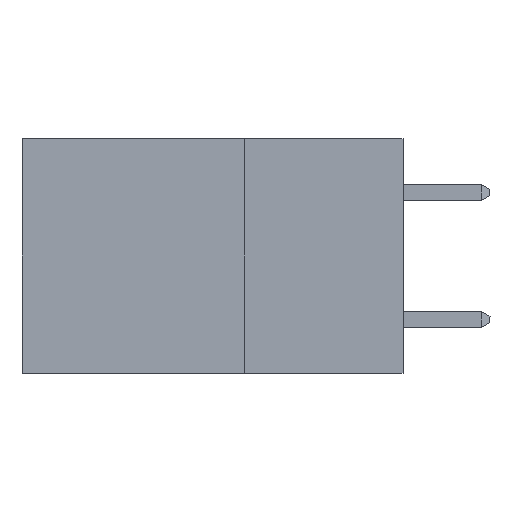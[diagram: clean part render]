
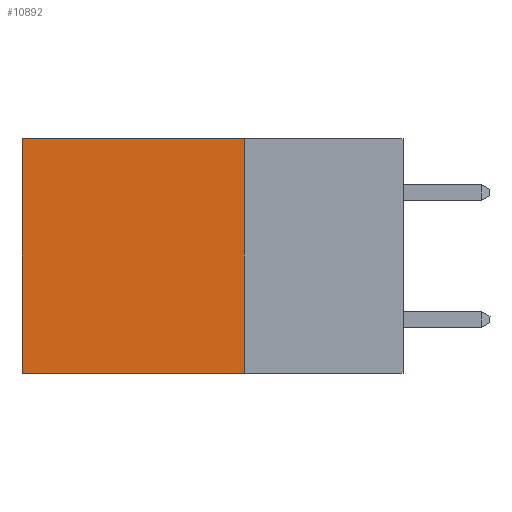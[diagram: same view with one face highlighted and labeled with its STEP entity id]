
A CAD part, left-side view. The second image highlights one B-rep face of the part: STEP entity #10892.
In plain terms, the highlighted planar face has unit normal (-1, 0, 0).
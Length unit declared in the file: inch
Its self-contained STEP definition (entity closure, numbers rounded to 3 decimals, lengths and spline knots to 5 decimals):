
#157 = ORIENTED_EDGE ( 'NONE', *, *, #10039, .F. ) ;
#158 = LINE ( 'NONE', #3170, #5974 ) ;
#489 = VERTEX_POINT ( 'NONE', #4031 ) ;
#647 = LINE ( 'NONE', #12323, #5846 ) ;
#1345 = DIRECTION ( 'NONE',  ( 0., 1., 0. ) ) ;
#1523 = CARTESIAN_POINT ( 'NONE',  ( 0.2875, 0.6, 0. ) ) ;
#1695 = VECTOR ( 'NONE', #12266, 39.37008 ) ;
#1858 = CARTESIAN_POINT ( 'NONE',  ( 0.2875, 0.25, 0. ) ) ;
#2393 = VECTOR ( 'NONE', #1345, 39.37008 ) ;
#2487 = VERTEX_POINT ( 'NONE', #4806 ) ;
#3170 = CARTESIAN_POINT ( 'NONE',  ( 0.2875, 0.25, 0. ) ) ;
#3178 = VERTEX_POINT ( 'NONE', #1523 ) ;
#3682 = ORIENTED_EDGE ( 'NONE', *, *, #5398, .T. ) ;
#3708 = DIRECTION ( 'NONE',  ( 1., 0., 0. ) ) ;
#4031 = CARTESIAN_POINT ( 'NONE',  ( 0.2875, 0.6, -0.37 ) ) ;
#4665 = FACE_OUTER_BOUND ( 'NONE', #6820, .T. ) ;
#4806 = CARTESIAN_POINT ( 'NONE',  ( 0.2875, 0.25, -0.37 ) ) ;
#5111 = LINE ( 'NONE', #10090, #2393 ) ;
#5174 = AXIS2_PLACEMENT_3D ( 'NONE', #1858, #3708, #7603 ) ;
#5203 = EDGE_CURVE ( 'NONE', #3178, #489, #647, .T. ) ;
#5398 = EDGE_CURVE ( 'NONE', #11629, #3178, #5111, .T. ) ;
#5846 = VECTOR ( 'NONE', #9459, 39.37008 ) ;
#5974 = VECTOR ( 'NONE', #12022, 39.37008 ) ;
#6820 = EDGE_LOOP ( 'NONE', ( #11789, #8402, #157, #3682 ) ) ;
#7603 = DIRECTION ( 'NONE',  ( 0., 0., -1. ) ) ;
#7640 = CARTESIAN_POINT ( 'NONE',  ( 0.2875, 0.25, 0. ) ) ;
#8402 = ORIENTED_EDGE ( 'NONE', *, *, #10255, .F. ) ;
#8555 = PLANE ( 'NONE',  #5174 ) ;
#9459 = DIRECTION ( 'NONE',  ( 0., 0., -1. ) ) ;
#9465 = CARTESIAN_POINT ( 'NONE',  ( 0.2875, 0.25, -0.37 ) ) ;
#10039 = EDGE_CURVE ( 'NONE', #11629, #2487, #158, .T. ) ;
#10090 = CARTESIAN_POINT ( 'NONE',  ( 0.2875, 0.25, 0. ) ) ;
#10255 = EDGE_CURVE ( 'NONE', #2487, #489, #11204, .T. ) ;
#10892 = ADVANCED_FACE ( 'NONE', ( #4665 ), #8555, .F. ) ;
#11204 = LINE ( 'NONE', #9465, #1695 ) ;
#11629 = VERTEX_POINT ( 'NONE', #7640 ) ;
#11789 = ORIENTED_EDGE ( 'NONE', *, *, #5203, .T. ) ;
#12022 = DIRECTION ( 'NONE',  ( 0., 0., -1. ) ) ;
#12266 = DIRECTION ( 'NONE',  ( 0., 1., 0. ) ) ;
#12323 = CARTESIAN_POINT ( 'NONE',  ( 0.2875, 0.6, 0. ) ) ;
